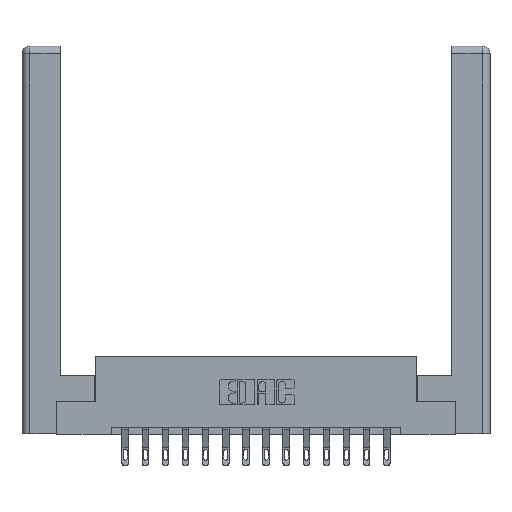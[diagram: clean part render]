
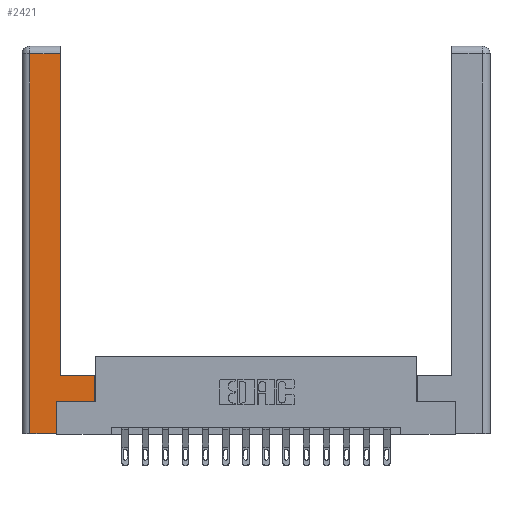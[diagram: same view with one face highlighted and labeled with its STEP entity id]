
A CAD part, top view. The second image highlights one B-rep face of the part: STEP entity #2421.
In plain terms, the highlighted planar face has unit normal (0, 0, 1).
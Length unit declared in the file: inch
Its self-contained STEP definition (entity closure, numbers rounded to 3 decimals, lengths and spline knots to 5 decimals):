
#235 = EDGE_LOOP ( 'NONE', ( #16474, #323, #4394, #17445, #9803, #1430, #15909, #12792 ) ) ;
#323 = ORIENTED_EDGE ( 'NONE', *, *, #9071, .T. ) ;
#674 = EDGE_CURVE ( 'NONE', #902, #4709, #9610, .T. ) ;
#902 = VERTEX_POINT ( 'NONE', #16820 ) ;
#1018 = CARTESIAN_POINT ( 'NONE',  ( 0.265, 0.245, 0. ) ) ;
#1034 = DIRECTION ( 'NONE',  ( -1., 0., 0. ) ) ;
#1055 = CARTESIAN_POINT ( 'NONE',  ( 0., 0., 0. ) ) ;
#1147 = CARTESIAN_POINT ( 'NONE',  ( 0.0615, 2.94, 0. ) ) ;
#1392 = CARTESIAN_POINT ( 'NONE',  ( 0.265, 0., 0. ) ) ;
#1430 = ORIENTED_EDGE ( 'NONE', *, *, #14057, .T. ) ;
#1498 = CARTESIAN_POINT ( 'NONE',  ( 0.0615, 0., 0. ) ) ;
#2135 = DIRECTION ( 'NONE',  ( 0., 0., -1. ) ) ;
#2421 = ADVANCED_FACE ( 'NONE', ( #15646 ), #17218, .F. ) ;
#3024 = CARTESIAN_POINT ( 'NONE',  ( 0.0615, 2.94, 0. ) ) ;
#3831 = VERTEX_POINT ( 'NONE', #9489 ) ;
#4229 = AXIS2_PLACEMENT_3D ( 'NONE', #1055, #2135, #15701 ) ;
#4278 = CARTESIAN_POINT ( 'NONE',  ( 0.565, 0.45, 0. ) ) ;
#4394 = ORIENTED_EDGE ( 'NONE', *, *, #13317, .T. ) ;
#4400 = DIRECTION ( 'NONE',  ( 0., -1., 0. ) ) ;
#4551 = DIRECTION ( 'NONE',  ( -1., 0., 0. ) ) ;
#4709 = VERTEX_POINT ( 'NONE', #15449 ) ;
#4970 = VECTOR ( 'NONE', #12978, 39.37008 ) ;
#4981 = EDGE_CURVE ( 'NONE', #3831, #14002, #11764, .T. ) ;
#5534 = LINE ( 'NONE', #11035, #13175 ) ;
#5920 = CARTESIAN_POINT ( 'NONE',  ( 0.565, 0.245, 0. ) ) ;
#6631 = CARTESIAN_POINT ( 'NONE',  ( 0.0615, 0., 0. ) ) ;
#6728 = DIRECTION ( 'NONE',  ( 0., 1., 0. ) ) ;
#6835 = VECTOR ( 'NONE', #14680, 39.37008 ) ;
#7095 = EDGE_CURVE ( 'NONE', #15153, #3831, #10420, .T. ) ;
#7402 = LINE ( 'NONE', #1498, #10346 ) ;
#8751 = VECTOR ( 'NONE', #4551, 39.37008 ) ;
#9071 = EDGE_CURVE ( 'NONE', #10874, #10791, #16241, .T. ) ;
#9489 = CARTESIAN_POINT ( 'NONE',  ( 0.265, 0., 0. ) ) ;
#9610 = LINE ( 'NONE', #13897, #8751 ) ;
#9803 = ORIENTED_EDGE ( 'NONE', *, *, #4981, .T. ) ;
#10197 = EDGE_CURVE ( 'NONE', #4709, #10874, #10517, .T. ) ;
#10232 = CARTESIAN_POINT ( 'NONE',  ( 0.265, 0.245, 0. ) ) ;
#10346 = VECTOR ( 'NONE', #4400, 39.37008 ) ;
#10420 = LINE ( 'NONE', #1392, #6835 ) ;
#10517 = LINE ( 'NONE', #14767, #14302 ) ;
#10537 = LINE ( 'NONE', #4278, #17244 ) ;
#10571 = VECTOR ( 'NONE', #1034, 39.37008 ) ;
#10791 = VERTEX_POINT ( 'NONE', #3024 ) ;
#10874 = VERTEX_POINT ( 'NONE', #16988 ) ;
#11035 = CARTESIAN_POINT ( 'NONE',  ( 0.565, 0.245, 0. ) ) ;
#11764 = LINE ( 'NONE', #10232, #4970 ) ;
#12792 = ORIENTED_EDGE ( 'NONE', *, *, #674, .T. ) ;
#12978 = DIRECTION ( 'NONE',  ( 0., 1., 0. ) ) ;
#13175 = VECTOR ( 'NONE', #13905, 39.37008 ) ;
#13317 = EDGE_CURVE ( 'NONE', #10791, #15153, #7402, .T. ) ;
#13897 = CARTESIAN_POINT ( 'NONE',  ( 0.295, 0.45, 0. ) ) ;
#13905 = DIRECTION ( 'NONE',  ( 1., 0., 0. ) ) ;
#14002 = VERTEX_POINT ( 'NONE', #1018 ) ;
#14057 = EDGE_CURVE ( 'NONE', #14002, #14724, #5534, .T. ) ;
#14302 = VECTOR ( 'NONE', #6728, 39.37008 ) ;
#14680 = DIRECTION ( 'NONE',  ( 1., 0., 0. ) ) ;
#14724 = VERTEX_POINT ( 'NONE', #5920 ) ;
#14767 = CARTESIAN_POINT ( 'NONE',  ( 0.295, 3., 0. ) ) ;
#15153 = VERTEX_POINT ( 'NONE', #6631 ) ;
#15449 = CARTESIAN_POINT ( 'NONE',  ( 0.295, 0.45, 0. ) ) ;
#15646 = FACE_OUTER_BOUND ( 'NONE', #235, .T. ) ;
#15701 = DIRECTION ( 'NONE',  ( -1., 0., 0. ) ) ;
#15909 = ORIENTED_EDGE ( 'NONE', *, *, #16184, .T. ) ;
#16184 = EDGE_CURVE ( 'NONE', #14724, #902, #10537, .T. ) ;
#16241 = LINE ( 'NONE', #1147, #10571 ) ;
#16474 = ORIENTED_EDGE ( 'NONE', *, *, #10197, .T. ) ;
#16654 = DIRECTION ( 'NONE',  ( 0., 1., 0. ) ) ;
#16820 = CARTESIAN_POINT ( 'NONE',  ( 0.565, 0.45, 0. ) ) ;
#16988 = CARTESIAN_POINT ( 'NONE',  ( 0.295, 2.94, 0. ) ) ;
#17218 = PLANE ( 'NONE',  #4229 ) ;
#17244 = VECTOR ( 'NONE', #16654, 39.37008 ) ;
#17445 = ORIENTED_EDGE ( 'NONE', *, *, #7095, .T. ) ;
